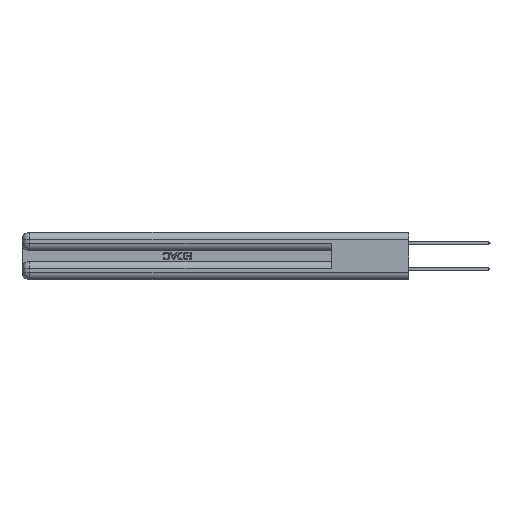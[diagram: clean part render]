
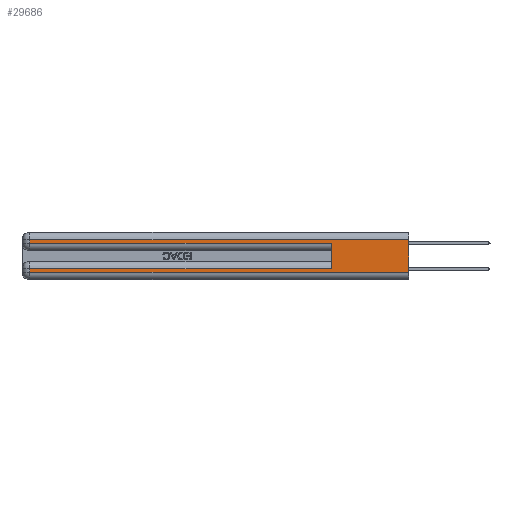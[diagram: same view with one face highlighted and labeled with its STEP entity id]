
A CAD part, left-side view. The second image highlights one B-rep face of the part: STEP entity #29686.
In plain terms, the highlighted planar face has unit normal (-1, 0, 0).
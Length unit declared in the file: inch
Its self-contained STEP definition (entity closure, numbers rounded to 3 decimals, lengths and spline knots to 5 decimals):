
#977 = VERTEX_POINT ( 'NONE', #27172 ) ;
#1120 = CARTESIAN_POINT ( 'NONE',  ( 0., 0., 0.37 ) ) ;
#1319 = ORIENTED_EDGE ( 'NONE', *, *, #5195, .T. ) ;
#1408 = DIRECTION ( 'NONE',  ( 0., 0., -1. ) ) ;
#1624 = DIRECTION ( 'NONE',  ( 0., -1., 0. ) ) ;
#2512 = DIRECTION ( 'NONE',  ( 0., 0., -1. ) ) ;
#4957 = DIRECTION ( 'NONE',  ( 0., 0., -1. ) ) ;
#5182 = LINE ( 'NONE', #32381, #23856 ) ;
#5195 = EDGE_CURVE ( 'NONE', #26917, #37080, #5182, .T. ) ;
#5639 = LINE ( 'NONE', #6516, #13310 ) ;
#6423 = EDGE_CURVE ( 'NONE', #26631, #16580, #5639, .T. ) ;
#6516 = CARTESIAN_POINT ( 'NONE',  ( 0., 0., 0.085 ) ) ;
#6997 = EDGE_CURVE ( 'NONE', #977, #23547, #38017, .T. ) ;
#8070 = VERTEX_POINT ( 'NONE', #11745 ) ;
#9066 = CARTESIAN_POINT ( 'NONE',  ( 0., 0., 0.31 ) ) ;
#9372 = VECTOR ( 'NONE', #33268, 39.37008 ) ;
#9497 = VECTOR ( 'NONE', #1408, 39.37008 ) ;
#11009 = CARTESIAN_POINT ( 'NONE',  ( 0., 0., 0.37 ) ) ;
#11500 = LINE ( 'NONE', #25042, #37421 ) ;
#11745 = CARTESIAN_POINT ( 'NONE',  ( 0., 0.6, 0.285 ) ) ;
#13137 = CARTESIAN_POINT ( 'NONE',  ( 0., 2.94, 0.37 ) ) ;
#13310 = VECTOR ( 'NONE', #25081, 39.37008 ) ;
#13680 = CARTESIAN_POINT ( 'NONE',  ( 0., 2.94, 0.285 ) ) ;
#14330 = AXIS2_PLACEMENT_3D ( 'NONE', #1120, #27239, #4957 ) ;
#15071 = ORIENTED_EDGE ( 'NONE', *, *, #6423, .T. ) ;
#15166 = CARTESIAN_POINT ( 'NONE',  ( 0., 0.6, 0.085 ) ) ;
#16580 = VERTEX_POINT ( 'NONE', #17726 ) ;
#17726 = CARTESIAN_POINT ( 'NONE',  ( 0., 2.94, 0.085 ) ) ;
#19401 = LINE ( 'NONE', #13137, #9497 ) ;
#20209 = ORIENTED_EDGE ( 'NONE', *, *, #6997, .T. ) ;
#20343 = CARTESIAN_POINT ( 'NONE',  ( 0., 0., 0.285 ) ) ;
#20426 = LINE ( 'NONE', #11009, #9372 ) ;
#20489 = VECTOR ( 'NONE', #1624, 39.37008 ) ;
#21267 = CARTESIAN_POINT ( 'NONE',  ( 0., 0., 0.06 ) ) ;
#22125 = CARTESIAN_POINT ( 'NONE',  ( 0., 2.94, 0.31 ) ) ;
#22549 = ORIENTED_EDGE ( 'NONE', *, *, #23289, .T. ) ;
#22775 = LINE ( 'NONE', #35018, #41093 ) ;
#23227 = ORIENTED_EDGE ( 'NONE', *, *, #28757, .F. ) ;
#23289 = EDGE_CURVE ( 'NONE', #31605, #8070, #30272, .T. ) ;
#23547 = VERTEX_POINT ( 'NONE', #22125 ) ;
#23566 = PLANE ( 'NONE',  #14330 ) ;
#23845 = ORIENTED_EDGE ( 'NONE', *, *, #31022, .T. ) ;
#23856 = VECTOR ( 'NONE', #39742, 39.37008 ) ;
#25042 = CARTESIAN_POINT ( 'NONE',  ( 0., 2.94, 0.37 ) ) ;
#25081 = DIRECTION ( 'NONE',  ( 0., 1., 0. ) ) ;
#26631 = VERTEX_POINT ( 'NONE', #15166 ) ;
#26917 = VERTEX_POINT ( 'NONE', #35058 ) ;
#27172 = CARTESIAN_POINT ( 'NONE',  ( 0., 0., 0.31 ) ) ;
#27239 = DIRECTION ( 'NONE',  ( 1., 0., 0. ) ) ;
#28475 = EDGE_CURVE ( 'NONE', #23547, #31605, #19401, .T. ) ;
#28757 = EDGE_CURVE ( 'NONE', #977, #37080, #20426, .T. ) ;
#29686 = ADVANCED_FACE ( 'NONE', ( #37555 ), #23566, .F. ) ;
#30272 = LINE ( 'NONE', #20343, #20489 ) ;
#31022 = EDGE_CURVE ( 'NONE', #16580, #26917, #11500, .T. ) ;
#31605 = VERTEX_POINT ( 'NONE', #13680 ) ;
#32381 = CARTESIAN_POINT ( 'NONE',  ( 0., 0., 0.06 ) ) ;
#33268 = DIRECTION ( 'NONE',  ( 0., 0., -1. ) ) ;
#34876 = DIRECTION ( 'NONE',  ( 0., 1., 0. ) ) ;
#35018 = CARTESIAN_POINT ( 'NONE',  ( 0., 0.6, 0.145 ) ) ;
#35058 = CARTESIAN_POINT ( 'NONE',  ( 0., 2.94, 0.06 ) ) ;
#37080 = VERTEX_POINT ( 'NONE', #21267 ) ;
#37421 = VECTOR ( 'NONE', #2512, 39.37008 ) ;
#37555 = FACE_OUTER_BOUND ( 'NONE', #41616, .T. ) ;
#38017 = LINE ( 'NONE', #9066, #47721 ) ;
#38688 = DIRECTION ( 'NONE',  ( 0., 0., 1. ) ) ;
#39570 = EDGE_CURVE ( 'NONE', #26631, #8070, #22775, .T. ) ;
#39742 = DIRECTION ( 'NONE',  ( 0., -1., 0. ) ) ;
#41093 = VECTOR ( 'NONE', #38688, 39.37008 ) ;
#41616 = EDGE_LOOP ( 'NONE', ( #23227, #20209, #43722, #22549, #47175, #15071, #23845, #1319 ) ) ;
#43722 = ORIENTED_EDGE ( 'NONE', *, *, #28475, .T. ) ;
#47175 = ORIENTED_EDGE ( 'NONE', *, *, #39570, .F. ) ;
#47721 = VECTOR ( 'NONE', #34876, 39.37008 ) ;
